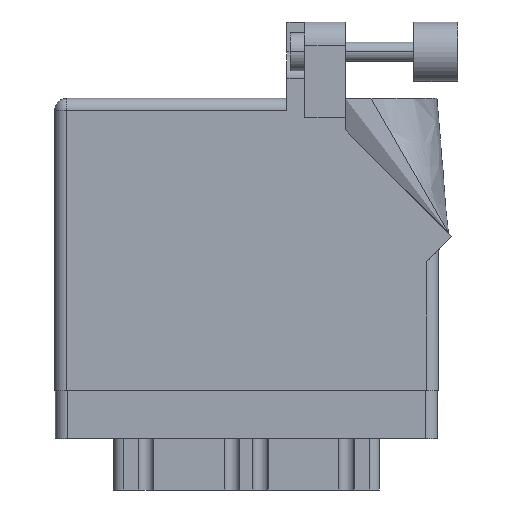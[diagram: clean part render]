
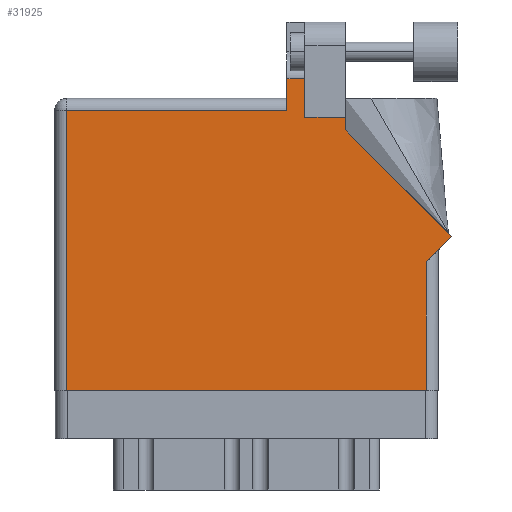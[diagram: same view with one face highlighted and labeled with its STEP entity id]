
A CAD part, front view. The second image highlights one B-rep face of the part: STEP entity #31925.
In plain terms, the highlighted face is planar.
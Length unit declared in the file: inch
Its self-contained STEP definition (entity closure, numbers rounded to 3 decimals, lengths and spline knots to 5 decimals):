
#38 = VECTOR ( 'NONE', #1829, 39.37008 ) ;
#1368 = AXIS2_PLACEMENT_3D ( 'NONE', #23696, #2606, #15901 ) ;
#1451 = VECTOR ( 'NONE', #9468, 39.37008 ) ;
#1572 = ORIENTED_EDGE ( 'NONE', *, *, #29094, .T. ) ;
#1639 = ORIENTED_EDGE ( 'NONE', *, *, #13417, .T. ) ;
#1829 = DIRECTION ( 'NONE',  ( -1., 0., 0. ) ) ;
#2193 = DIRECTION ( 'NONE',  ( 1., 0., 0. ) ) ;
#2470 = ORIENTED_EDGE ( 'NONE', *, *, #9787, .T. ) ;
#2604 = CARTESIAN_POINT ( 'NONE',  ( 1.948, 0.675, 0. ) ) ;
#2606 = DIRECTION ( 'NONE',  ( 0., 0., -1. ) ) ;
#2620 = EDGE_CURVE ( 'NONE', #25024, #12468, #22581, .T. ) ;
#3062 = VECTOR ( 'NONE', #18031, 39.37008 ) ;
#3540 = LINE ( 'NONE', #4249, #10299 ) ;
#3547 = LINE ( 'NONE', #30447, #6998 ) ;
#4249 = CARTESIAN_POINT ( 'NONE',  ( 1.64177, 1.6315, 0. ) ) ;
#5663 = VERTEX_POINT ( 'NONE', #2604 ) ;
#5963 = VERTEX_POINT ( 'NONE', #26839 ) ;
#6588 = CARTESIAN_POINT ( 'NONE',  ( 2.08071, 0.80771, 0. ) ) ;
#6722 = DIRECTION ( 'NONE',  ( -1., 0., 0. ) ) ;
#6998 = VECTOR ( 'NONE', #24983, 39.37008 ) ;
#7212 = EDGE_CURVE ( 'NONE', #5963, #5663, #18355, .T. ) ;
#7351 = VERTEX_POINT ( 'NONE', #32285 ) ;
#8084 = VECTOR ( 'NONE', #8577, 39.37008 ) ;
#8577 = DIRECTION ( 'NONE',  ( -0.707, 0.707, 0. ) ) ;
#9352 = CARTESIAN_POINT ( 'NONE',  ( 1.524, 1.36442, 0. ) ) ;
#9468 = DIRECTION ( 'NONE',  ( 0., -1., 0. ) ) ;
#9787 = EDGE_CURVE ( 'NONE', #23921, #7351, #28705, .T. ) ;
#9806 = LINE ( 'NONE', #20638, #33892 ) ;
#10202 = ORIENTED_EDGE ( 'NONE', *, *, #26799, .T. ) ;
#10299 = VECTOR ( 'NONE', #6722, 39.37008 ) ;
#11047 = VECTOR ( 'NONE', #12327, 39.37008 ) ;
#12327 = DIRECTION ( 'NONE',  ( 0., 1., 0. ) ) ;
#12468 = VERTEX_POINT ( 'NONE', #15499 ) ;
#12537 = CARTESIAN_POINT ( 'NONE',  ( 1.217, 1.53, 0. ) ) ;
#12859 = CARTESIAN_POINT ( 'NONE',  ( 0.062, 1.468, 0. ) ) ;
#13417 = EDGE_CURVE ( 'NONE', #5663, #23719, #31656, .T. ) ;
#14110 = CARTESIAN_POINT ( 'NONE',  ( 1.311, 1.6315, 0. ) ) ;
#15066 = LINE ( 'NONE', #34665, #27292 ) ;
#15499 = CARTESIAN_POINT ( 'NONE',  ( 0.062, 0., 0. ) ) ;
#15590 = ORIENTED_EDGE ( 'NONE', *, *, #30054, .T. ) ;
#15901 = DIRECTION ( 'NONE',  ( -1., 0., 0. ) ) ;
#16104 = CARTESIAN_POINT ( 'NONE',  ( 2.01, 0.737, 0. ) ) ;
#16912 = CARTESIAN_POINT ( 'NONE',  ( 1.217, 1.468, 0. ) ) ;
#17965 = CARTESIAN_POINT ( 'NONE',  ( 1.524, 1.43, 0. ) ) ;
#18031 = DIRECTION ( 'NONE',  ( 0., -1., 0. ) ) ;
#18102 = VERTEX_POINT ( 'NONE', #16912 ) ;
#18276 = EDGE_CURVE ( 'NONE', #12468, #5963, #9806, .T. ) ;
#18355 = LINE ( 'NONE', #21005, #11047 ) ;
#20036 = LINE ( 'NONE', #12537, #3062 ) ;
#20254 = VERTEX_POINT ( 'NONE', #14110 ) ;
#20461 = CARTESIAN_POINT ( 'NONE',  ( 0.062, 0., 0. ) ) ;
#20638 = CARTESIAN_POINT ( 'NONE',  ( 0., 0., 0. ) ) ;
#21005 = CARTESIAN_POINT ( 'NONE',  ( 1.948, 0.737, 0. ) ) ;
#21065 = VERTEX_POINT ( 'NONE', #27784 ) ;
#21174 = ORIENTED_EDGE ( 'NONE', *, *, #7212, .T. ) ;
#21312 = VERTEX_POINT ( 'NONE', #35000 ) ;
#21788 = EDGE_LOOP ( 'NONE', ( #28521, #34692, #15590, #29359, #34515, #24073, #21174, #1639, #1572, #2470, #10202 ) ) ;
#22581 = LINE ( 'NONE', #20461, #1451 ) ;
#23202 = DIRECTION ( 'NONE',  ( -1., 0., 0. ) ) ;
#23696 = CARTESIAN_POINT ( 'NONE',  ( 0., 1.53, 0. ) ) ;
#23719 = VERTEX_POINT ( 'NONE', #6588 ) ;
#23921 = VERTEX_POINT ( 'NONE', #9352 ) ;
#24073 = ORIENTED_EDGE ( 'NONE', *, *, #18276, .T. ) ;
#24515 = VECTOR ( 'NONE', #25886, 39.37008 ) ;
#24896 = CARTESIAN_POINT ( 'NONE',  ( 2.08071, 0.80771, 0. ) ) ;
#24983 = DIRECTION ( 'NONE',  ( 0., 1., 0. ) ) ;
#25024 = VERTEX_POINT ( 'NONE', #12859 ) ;
#25886 = DIRECTION ( 'NONE',  ( 0., 1., 0. ) ) ;
#26794 = VECTOR ( 'NONE', #29017, 39.37008 ) ;
#26799 = EDGE_CURVE ( 'NONE', #7351, #21312, #34042, .T. ) ;
#26839 = CARTESIAN_POINT ( 'NONE',  ( 1.948, 0., 0. ) ) ;
#27292 = VECTOR ( 'NONE', #23202, 39.37008 ) ;
#27784 = CARTESIAN_POINT ( 'NONE',  ( 1.217, 1.6315, 0. ) ) ;
#28282 = EDGE_CURVE ( 'NONE', #20254, #21065, #3540, .T. ) ;
#28388 = EDGE_CURVE ( 'NONE', #18102, #25024, #15066, .T. ) ;
#28521 = ORIENTED_EDGE ( 'NONE', *, *, #30017, .T. ) ;
#28705 = LINE ( 'NONE', #28877, #24515 ) ;
#28877 = CARTESIAN_POINT ( 'NONE',  ( 1.524, 1.36442, 0. ) ) ;
#29017 = DIRECTION ( 'NONE',  ( 0.707, 0.707, 0. ) ) ;
#29094 = EDGE_CURVE ( 'NONE', #23719, #23921, #33530, .T. ) ;
#29359 = ORIENTED_EDGE ( 'NONE', *, *, #28388, .T. ) ;
#30017 = EDGE_CURVE ( 'NONE', #21312, #20254, #3547, .T. ) ;
#30054 = EDGE_CURVE ( 'NONE', #21065, #18102, #20036, .T. ) ;
#30447 = CARTESIAN_POINT ( 'NONE',  ( 1.311, 1.43, 0. ) ) ;
#31629 = FACE_OUTER_BOUND ( 'NONE', #21788, .T. ) ;
#31656 = LINE ( 'NONE', #16104, #26794 ) ;
#31925 = ADVANCED_FACE ( 'NONE', ( #31629 ), #32156, .F. ) ;
#32156 = PLANE ( 'NONE',  #1368 ) ;
#32285 = CARTESIAN_POINT ( 'NONE',  ( 1.524, 1.43, 0. ) ) ;
#33530 = LINE ( 'NONE', #24896, #8084 ) ;
#33892 = VECTOR ( 'NONE', #2193, 39.37008 ) ;
#34042 = LINE ( 'NONE', #17965, #38 ) ;
#34515 = ORIENTED_EDGE ( 'NONE', *, *, #2620, .T. ) ;
#34665 = CARTESIAN_POINT ( 'NONE',  ( 0., 1.468, 0. ) ) ;
#34692 = ORIENTED_EDGE ( 'NONE', *, *, #28282, .T. ) ;
#35000 = CARTESIAN_POINT ( 'NONE',  ( 1.311, 1.43, 0. ) ) ;
